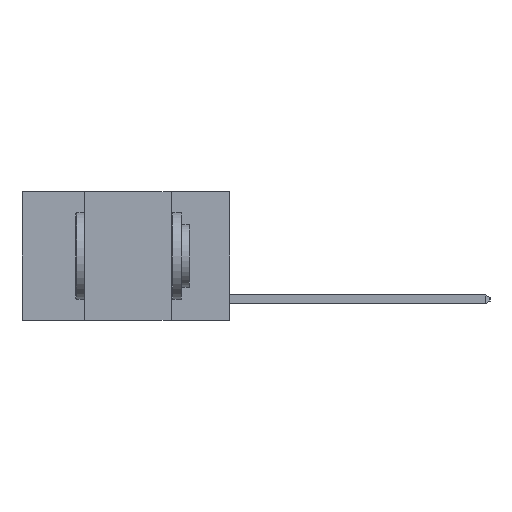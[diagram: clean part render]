
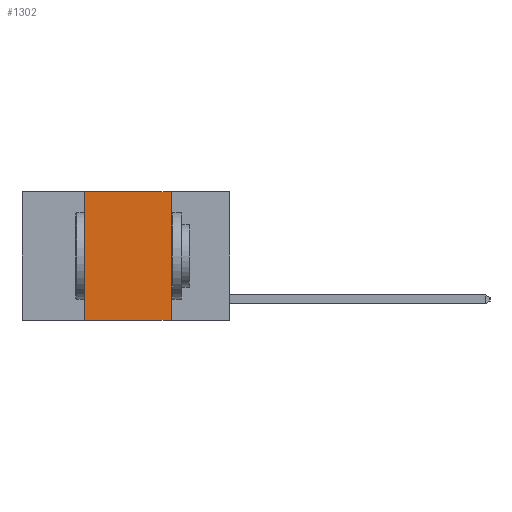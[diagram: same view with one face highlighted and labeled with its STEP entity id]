
A CAD part, left-side view. The second image highlights one B-rep face of the part: STEP entity #1302.
In plain terms, the highlighted planar face has unit normal (-1, 0, 0).
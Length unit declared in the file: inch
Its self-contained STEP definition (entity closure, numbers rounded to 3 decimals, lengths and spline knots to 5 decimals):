
#282 = DIRECTION ( 'NONE',  ( 1., 0., 0. ) ) ;
#815 = VERTEX_POINT ( 'NONE', #11433 ) ;
#1016 = ORIENTED_EDGE ( 'NONE', *, *, #9450, .F. ) ;
#1302 = ADVANCED_FACE ( 'NONE', ( #11368 ), #5021, .F. ) ;
#2048 = AXIS2_PLACEMENT_3D ( 'NONE', #4115, #282, #6793 ) ;
#2060 = VECTOR ( 'NONE', #8314, 39.37008 ) ;
#2224 = LINE ( 'NONE', #4694, #4310 ) ;
#2731 = VERTEX_POINT ( 'NONE', #3666 ) ;
#3100 = EDGE_CURVE ( 'NONE', #815, #4332, #11314, .T. ) ;
#3530 = ORIENTED_EDGE ( 'NONE', *, *, #4400, .F. ) ;
#3666 = CARTESIAN_POINT ( 'NONE',  ( 0., 0.17, 0. ) ) ;
#3944 = DIRECTION ( 'NONE',  ( 0., 0., -1. ) ) ;
#4115 = CARTESIAN_POINT ( 'NONE',  ( 0., 0.6, 0. ) ) ;
#4310 = VECTOR ( 'NONE', #11765, 39.37008 ) ;
#4332 = VERTEX_POINT ( 'NONE', #6322 ) ;
#4400 = EDGE_CURVE ( 'NONE', #11680, #2731, #2224, .T. ) ;
#4694 = CARTESIAN_POINT ( 'NONE',  ( 0., 0.6, 0. ) ) ;
#5005 = DIRECTION ( 'NONE',  ( 0., -1., 0. ) ) ;
#5021 = PLANE ( 'NONE',  #2048 ) ;
#5266 = EDGE_CURVE ( 'NONE', #815, #11680, #8903, .T. ) ;
#5765 = LINE ( 'NONE', #7493, #9964 ) ;
#5900 = ORIENTED_EDGE ( 'NONE', *, *, #5266, .F. ) ;
#6322 = CARTESIAN_POINT ( 'NONE',  ( 0., 0.17, -0.37 ) ) ;
#6482 = EDGE_LOOP ( 'NONE', ( #1016, #3530, #5900, #10633 ) ) ;
#6793 = DIRECTION ( 'NONE',  ( 0., 0., -1. ) ) ;
#7431 = CARTESIAN_POINT ( 'NONE',  ( 0., 0.42, 0. ) ) ;
#7493 = CARTESIAN_POINT ( 'NONE',  ( 0., 0.17, 0. ) ) ;
#7642 = CARTESIAN_POINT ( 'NONE',  ( 0., 0.6, -0.37 ) ) ;
#8209 = CARTESIAN_POINT ( 'NONE',  ( 0., 0.42, 0. ) ) ;
#8314 = DIRECTION ( 'NONE',  ( 0., 0., 1. ) ) ;
#8903 = LINE ( 'NONE', #7431, #2060 ) ;
#8970 = VECTOR ( 'NONE', #5005, 39.37008 ) ;
#9450 = EDGE_CURVE ( 'NONE', #2731, #4332, #5765, .T. ) ;
#9964 = VECTOR ( 'NONE', #3944, 39.37008 ) ;
#10633 = ORIENTED_EDGE ( 'NONE', *, *, #3100, .T. ) ;
#11314 = LINE ( 'NONE', #7642, #8970 ) ;
#11368 = FACE_OUTER_BOUND ( 'NONE', #6482, .T. ) ;
#11433 = CARTESIAN_POINT ( 'NONE',  ( 0., 0.42, -0.37 ) ) ;
#11680 = VERTEX_POINT ( 'NONE', #8209 ) ;
#11765 = DIRECTION ( 'NONE',  ( 0., -1., 0. ) ) ;
